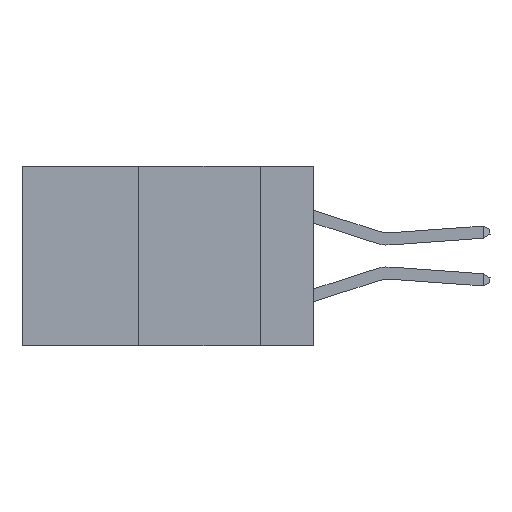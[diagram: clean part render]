
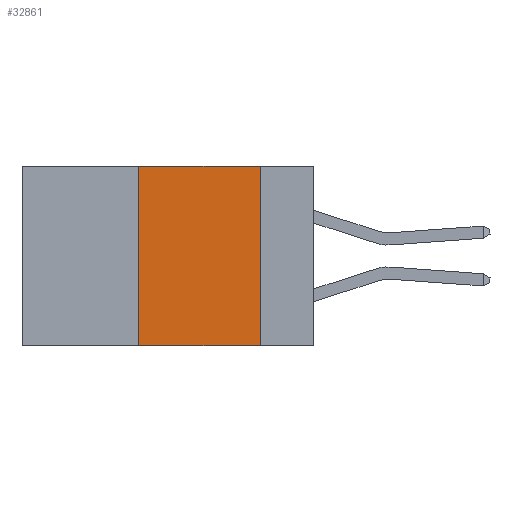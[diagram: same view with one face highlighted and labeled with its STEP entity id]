
A CAD part, left-side view. The second image highlights one B-rep face of the part: STEP entity #32861.
In plain terms, the highlighted planar face has unit normal (-1, 0, 0).
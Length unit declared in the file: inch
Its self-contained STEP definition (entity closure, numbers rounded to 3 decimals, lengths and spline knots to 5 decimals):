
#79 = ORIENTED_EDGE ( 'NONE', *, *, #37398, .F. ) ;
#500 = AXIS2_PLACEMENT_3D ( 'NONE', #8051, #23077, #7909 ) ;
#2514 = VECTOR ( 'NONE', #5559, 39.37008 ) ;
#3611 = VECTOR ( 'NONE', #15053, 39.37008 ) ;
#4098 = EDGE_LOOP ( 'NONE', ( #27223, #79, #31309, #17754 ) ) ;
#4184 = VERTEX_POINT ( 'NONE', #6453 ) ;
#4552 = PLANE ( 'NONE',  #500 ) ;
#5559 = DIRECTION ( 'NONE',  ( 0., -1., 0. ) ) ;
#6453 = CARTESIAN_POINT ( 'NONE',  ( 0., 0.11, 0. ) ) ;
#7909 = DIRECTION ( 'NONE',  ( 0., 0., -1. ) ) ;
#8051 = CARTESIAN_POINT ( 'NONE',  ( 0., 0.6, 0. ) ) ;
#8445 = EDGE_CURVE ( 'NONE', #4184, #8715, #33393, .T. ) ;
#8715 = VERTEX_POINT ( 'NONE', #11000 ) ;
#11000 = CARTESIAN_POINT ( 'NONE',  ( 0., 0.11, -0.37 ) ) ;
#14289 = LINE ( 'NONE', #30066, #3611 ) ;
#15053 = DIRECTION ( 'NONE',  ( 0., -1., 0. ) ) ;
#16603 = VECTOR ( 'NONE', #19306, 39.37008 ) ;
#16896 = EDGE_CURVE ( 'NONE', #31600, #8715, #14289, .T. ) ;
#17754 = ORIENTED_EDGE ( 'NONE', *, *, #16896, .T. ) ;
#18042 = EDGE_CURVE ( 'NONE', #31600, #36905, #29499, .T. ) ;
#18882 = CARTESIAN_POINT ( 'NONE',  ( 0., 0.36, 0. ) ) ;
#19306 = DIRECTION ( 'NONE',  ( 0., 0., -1. ) ) ;
#22586 = FACE_OUTER_BOUND ( 'NONE', #4098, .T. ) ;
#23077 = DIRECTION ( 'NONE',  ( 1., 0., 0. ) ) ;
#27223 = ORIENTED_EDGE ( 'NONE', *, *, #8445, .F. ) ;
#28679 = CARTESIAN_POINT ( 'NONE',  ( 0., 0.11, 0. ) ) ;
#29499 = LINE ( 'NONE', #34421, #37659 ) ;
#30066 = CARTESIAN_POINT ( 'NONE',  ( 0., 0.6, -0.37 ) ) ;
#30158 = CARTESIAN_POINT ( 'NONE',  ( 0., 0.6, 0. ) ) ;
#31309 = ORIENTED_EDGE ( 'NONE', *, *, #18042, .F. ) ;
#31600 = VERTEX_POINT ( 'NONE', #36828 ) ;
#32861 = ADVANCED_FACE ( 'NONE', ( #22586 ), #4552, .F. ) ;
#33393 = LINE ( 'NONE', #28679, #16603 ) ;
#34421 = CARTESIAN_POINT ( 'NONE',  ( 0., 0.36, 0. ) ) ;
#34688 = DIRECTION ( 'NONE',  ( 0., 0., 1. ) ) ;
#36111 = LINE ( 'NONE', #30158, #2514 ) ;
#36828 = CARTESIAN_POINT ( 'NONE',  ( 0., 0.36, -0.37 ) ) ;
#36905 = VERTEX_POINT ( 'NONE', #18882 ) ;
#37398 = EDGE_CURVE ( 'NONE', #36905, #4184, #36111, .T. ) ;
#37659 = VECTOR ( 'NONE', #34688, 39.37008 ) ;
